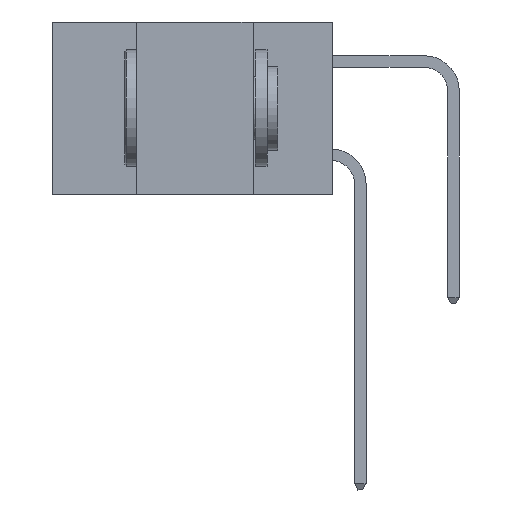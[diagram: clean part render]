
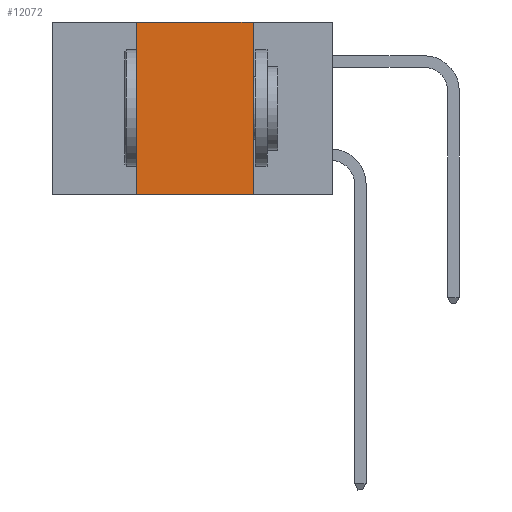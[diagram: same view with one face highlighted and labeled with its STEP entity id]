
A CAD part, left-side view. The second image highlights one B-rep face of the part: STEP entity #12072.
In plain terms, the highlighted planar face has unit normal (-1, 0, 0).
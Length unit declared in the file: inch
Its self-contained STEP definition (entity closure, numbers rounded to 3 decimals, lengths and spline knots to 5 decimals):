
#427 = EDGE_CURVE ( 'NONE', #21258, #3123, #22273, .T. ) ;
#1215 = CARTESIAN_POINT ( 'NONE',  ( 0., 0.42, -0.37 ) ) ;
#2030 = DIRECTION ( 'NONE',  ( 0., 0., -1. ) ) ;
#2548 = CARTESIAN_POINT ( 'NONE',  ( 0., 0.6, -0.37 ) ) ;
#3089 = EDGE_CURVE ( 'NONE', #3123, #11916, #10403, .T. ) ;
#3093 = FACE_OUTER_BOUND ( 'NONE', #14970, .T. ) ;
#3123 = VERTEX_POINT ( 'NONE', #21005 ) ;
#3332 = VECTOR ( 'NONE', #8391, 39.37008 ) ;
#4401 = EDGE_CURVE ( 'NONE', #11916, #6565, #20588, .T. ) ;
#4472 = ORIENTED_EDGE ( 'NONE', *, *, #21738, .T. ) ;
#5821 = AXIS2_PLACEMENT_3D ( 'NONE', #21371, #13716, #2030 ) ;
#6565 = VERTEX_POINT ( 'NONE', #7584 ) ;
#7584 = CARTESIAN_POINT ( 'NONE',  ( 0., 0.17, -0.37 ) ) ;
#7939 = LINE ( 'NONE', #2548, #3332 ) ;
#8391 = DIRECTION ( 'NONE',  ( 0., -1., 0. ) ) ;
#9728 = DIRECTION ( 'NONE',  ( 0., 0., 1. ) ) ;
#10403 = LINE ( 'NONE', #22847, #20047 ) ;
#11298 = CARTESIAN_POINT ( 'NONE',  ( 0., 0.17, 0. ) ) ;
#11467 = VECTOR ( 'NONE', #9728, 39.37008 ) ;
#11916 = VERTEX_POINT ( 'NONE', #11298 ) ;
#12072 = ADVANCED_FACE ( 'NONE', ( #3093 ), #23257, .F. ) ;
#12996 = ORIENTED_EDGE ( 'NONE', *, *, #4401, .F. ) ;
#13716 = DIRECTION ( 'NONE',  ( 1., 0., 0. ) ) ;
#14970 = EDGE_LOOP ( 'NONE', ( #12996, #18718, #19327, #4472 ) ) ;
#16078 = CARTESIAN_POINT ( 'NONE',  ( 0., 0.17, -0.37 ) ) ;
#18718 = ORIENTED_EDGE ( 'NONE', *, *, #3089, .F. ) ;
#18874 = CARTESIAN_POINT ( 'NONE',  ( 0., 0.42, -0.37 ) ) ;
#19327 = ORIENTED_EDGE ( 'NONE', *, *, #427, .F. ) ;
#19942 = DIRECTION ( 'NONE',  ( 0., 0., -1. ) ) ;
#19969 = VECTOR ( 'NONE', #19942, 39.37008 ) ;
#20047 = VECTOR ( 'NONE', #23339, 39.37008 ) ;
#20588 = LINE ( 'NONE', #16078, #19969 ) ;
#21005 = CARTESIAN_POINT ( 'NONE',  ( 0., 0.42, 0. ) ) ;
#21258 = VERTEX_POINT ( 'NONE', #1215 ) ;
#21371 = CARTESIAN_POINT ( 'NONE',  ( 0., 0.6, 0. ) ) ;
#21738 = EDGE_CURVE ( 'NONE', #21258, #6565, #7939, .T. ) ;
#22273 = LINE ( 'NONE', #18874, #11467 ) ;
#22847 = CARTESIAN_POINT ( 'NONE',  ( 0., 0.6, 0. ) ) ;
#23257 = PLANE ( 'NONE',  #5821 ) ;
#23339 = DIRECTION ( 'NONE',  ( 0., -1., 0. ) ) ;
